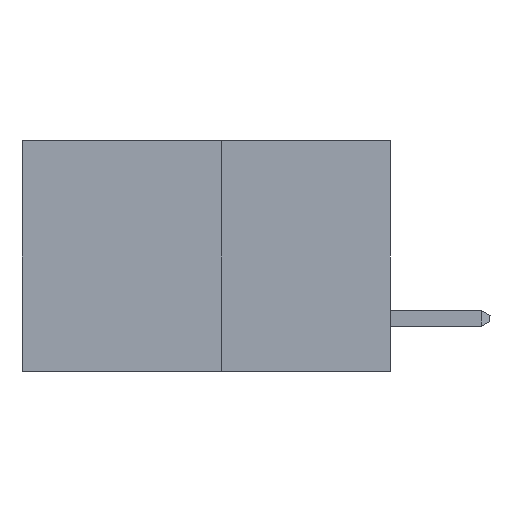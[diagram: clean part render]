
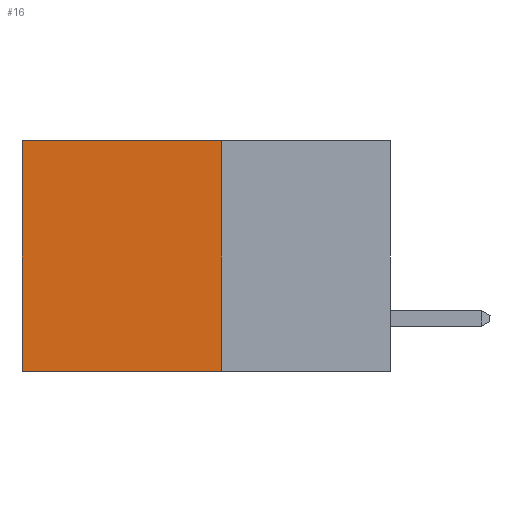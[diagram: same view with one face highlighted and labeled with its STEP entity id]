
A CAD part, left-side view. The second image highlights one B-rep face of the part: STEP entity #16.
In plain terms, the highlighted planar face has unit normal (-1, 0, 0).
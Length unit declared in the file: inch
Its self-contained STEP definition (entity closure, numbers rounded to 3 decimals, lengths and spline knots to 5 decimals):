
#16 = ADVANCED_FACE ( 'NONE', ( #4021 ), #979, .F. ) ;
#730 = ORIENTED_EDGE ( 'NONE', *, *, #6270, .T. ) ;
#901 = LINE ( 'NONE', #6327, #8450 ) ;
#979 = PLANE ( 'NONE',  #7327 ) ;
#1408 = LINE ( 'NONE', #7473, #6385 ) ;
#2436 = DIRECTION ( 'NONE',  ( 1., 0., 0. ) ) ;
#2445 = ORIENTED_EDGE ( 'NONE', *, *, #6694, .F. ) ;
#3282 = CARTESIAN_POINT ( 'NONE',  ( 0.277, 0.59, -0.37 ) ) ;
#3360 = ORIENTED_EDGE ( 'NONE', *, *, #9948, .F. ) ;
#3648 = LINE ( 'NONE', #4384, #8821 ) ;
#3719 = VERTEX_POINT ( 'NONE', #5248 ) ;
#4021 = FACE_OUTER_BOUND ( 'NONE', #11048, .T. ) ;
#4384 = CARTESIAN_POINT ( 'NONE',  ( 0.277, 0.27, 0. ) ) ;
#4694 = CARTESIAN_POINT ( 'NONE',  ( 0.277, 0.27, -0.37 ) ) ;
#4695 = DIRECTION ( 'NONE',  ( 0., 1., 0. ) ) ;
#5147 = ORIENTED_EDGE ( 'NONE', *, *, #7292, .T. ) ;
#5248 = CARTESIAN_POINT ( 'NONE',  ( 0.277, 0.27, 0. ) ) ;
#6270 = EDGE_CURVE ( 'NONE', #3719, #7114, #3648, .T. ) ;
#6327 = CARTESIAN_POINT ( 'NONE',  ( 0.277, 0.27, -0.37 ) ) ;
#6335 = CARTESIAN_POINT ( 'NONE',  ( 0.277, 0.59, 0. ) ) ;
#6368 = DIRECTION ( 'NONE',  ( 0., 1., 0. ) ) ;
#6385 = VECTOR ( 'NONE', #7430, 39.37008 ) ;
#6694 = EDGE_CURVE ( 'NONE', #3719, #11930, #11352, .T. ) ;
#7114 = VERTEX_POINT ( 'NONE', #6335 ) ;
#7292 = EDGE_CURVE ( 'NONE', #7114, #11813, #1408, .T. ) ;
#7327 = AXIS2_PLACEMENT_3D ( 'NONE', #12506, #2436, #12402 ) ;
#7430 = DIRECTION ( 'NONE',  ( 0., 0., -1. ) ) ;
#7473 = CARTESIAN_POINT ( 'NONE',  ( 0.277, 0.59, -0.37 ) ) ;
#8450 = VECTOR ( 'NONE', #6368, 39.37008 ) ;
#8821 = VECTOR ( 'NONE', #4695, 39.37008 ) ;
#9948 = EDGE_CURVE ( 'NONE', #11930, #11813, #901, .T. ) ;
#11048 = EDGE_LOOP ( 'NONE', ( #5147, #3360, #2445, #730 ) ) ;
#11072 = VECTOR ( 'NONE', #11878, 39.37008 ) ;
#11352 = LINE ( 'NONE', #12241, #11072 ) ;
#11813 = VERTEX_POINT ( 'NONE', #3282 ) ;
#11878 = DIRECTION ( 'NONE',  ( 0., 0., -1. ) ) ;
#11930 = VERTEX_POINT ( 'NONE', #4694 ) ;
#12241 = CARTESIAN_POINT ( 'NONE',  ( 0.277, 0.27, -0.37 ) ) ;
#12402 = DIRECTION ( 'NONE',  ( 0., 0., -1. ) ) ;
#12506 = CARTESIAN_POINT ( 'NONE',  ( 0.277, 0.27, -0.37 ) ) ;
